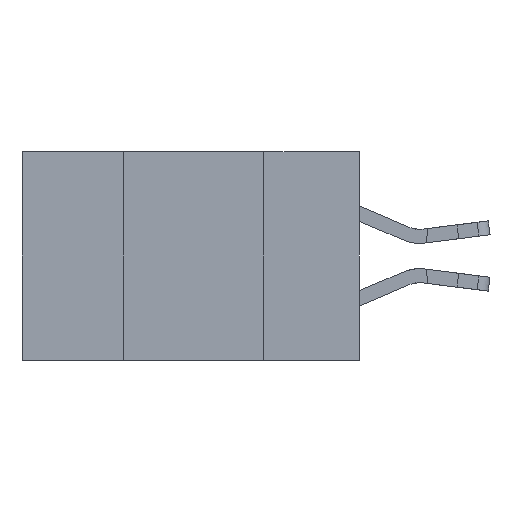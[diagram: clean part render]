
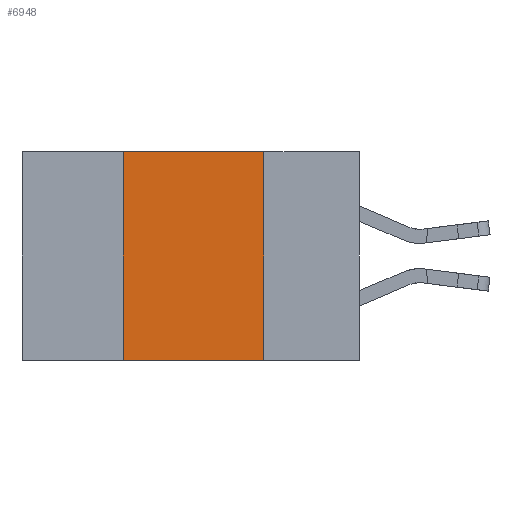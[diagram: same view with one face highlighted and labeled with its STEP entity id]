
A CAD part, left-side view. The second image highlights one B-rep face of the part: STEP entity #6948.
In plain terms, the highlighted planar face has unit normal (-1, 0, 0).
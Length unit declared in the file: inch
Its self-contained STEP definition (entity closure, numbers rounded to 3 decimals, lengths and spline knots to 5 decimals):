
#770 = VERTEX_POINT ( 'NONE', #2301 ) ;
#1649 = VERTEX_POINT ( 'NONE', #6435 ) ;
#2301 = CARTESIAN_POINT ( 'NONE',  ( 0., 0.17, -0.37 ) ) ;
#4230 = EDGE_CURVE ( 'NONE', #1649, #770, #6939, .T. ) ;
#4449 = EDGE_LOOP ( 'NONE', ( #28553, #10762, #10497, #5113 ) ) ;
#4470 = DIRECTION ( 'NONE',  ( 0., -1., 0. ) ) ;
#5113 = ORIENTED_EDGE ( 'NONE', *, *, #12426, .T. ) ;
#5343 = CARTESIAN_POINT ( 'NONE',  ( 0., 0.17, 0. ) ) ;
#5449 = VECTOR ( 'NONE', #26309, 39.37008 ) ;
#5538 = FACE_OUTER_BOUND ( 'NONE', #4449, .T. ) ;
#6435 = CARTESIAN_POINT ( 'NONE',  ( 0., 0.17, 0. ) ) ;
#6648 = LINE ( 'NONE', #22033, #23911 ) ;
#6939 = LINE ( 'NONE', #5343, #14479 ) ;
#6948 = ADVANCED_FACE ( 'NONE', ( #5538 ), #14349, .F. ) ;
#8069 = CARTESIAN_POINT ( 'NONE',  ( 0., 0.6, 0. ) ) ;
#9153 = CARTESIAN_POINT ( 'NONE',  ( 0., 0.42, -0.37 ) ) ;
#9626 = AXIS2_PLACEMENT_3D ( 'NONE', #21060, #18413, #18134 ) ;
#10497 = ORIENTED_EDGE ( 'NONE', *, *, #13395, .F. ) ;
#10762 = ORIENTED_EDGE ( 'NONE', *, *, #15810, .F. ) ;
#12426 = EDGE_CURVE ( 'NONE', #27783, #770, #6648, .T. ) ;
#13395 = EDGE_CURVE ( 'NONE', #27783, #14326, #22373, .T. ) ;
#14326 = VERTEX_POINT ( 'NONE', #25302 ) ;
#14349 = PLANE ( 'NONE',  #9626 ) ;
#14479 = VECTOR ( 'NONE', #23031, 39.37008 ) ;
#15144 = LINE ( 'NONE', #8069, #19343 ) ;
#15810 = EDGE_CURVE ( 'NONE', #14326, #1649, #15144, .T. ) ;
#18134 = DIRECTION ( 'NONE',  ( 0., 0., -1. ) ) ;
#18413 = DIRECTION ( 'NONE',  ( 1., 0., 0. ) ) ;
#19343 = VECTOR ( 'NONE', #19361, 39.37008 ) ;
#19361 = DIRECTION ( 'NONE',  ( 0., -1., 0. ) ) ;
#20193 = CARTESIAN_POINT ( 'NONE',  ( 0., 0.42, 0. ) ) ;
#21060 = CARTESIAN_POINT ( 'NONE',  ( 0., 0.6, 0. ) ) ;
#22033 = CARTESIAN_POINT ( 'NONE',  ( 0., 0.6, -0.37 ) ) ;
#22373 = LINE ( 'NONE', #20193, #5449 ) ;
#23031 = DIRECTION ( 'NONE',  ( 0., 0., -1. ) ) ;
#23911 = VECTOR ( 'NONE', #4470, 39.37008 ) ;
#25302 = CARTESIAN_POINT ( 'NONE',  ( 0., 0.42, 0. ) ) ;
#26309 = DIRECTION ( 'NONE',  ( 0., 0., 1. ) ) ;
#27783 = VERTEX_POINT ( 'NONE', #9153 ) ;
#28553 = ORIENTED_EDGE ( 'NONE', *, *, #4230, .F. ) ;
